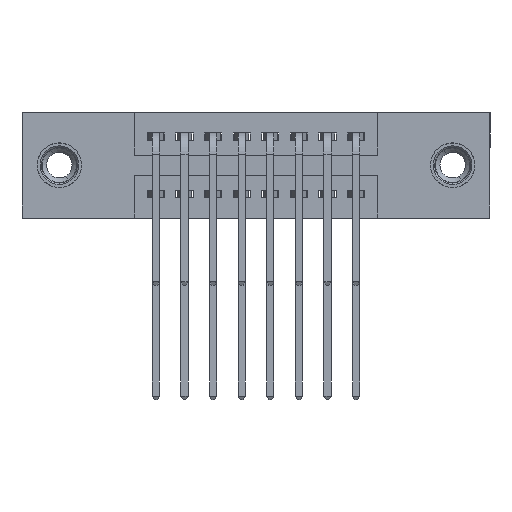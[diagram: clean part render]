
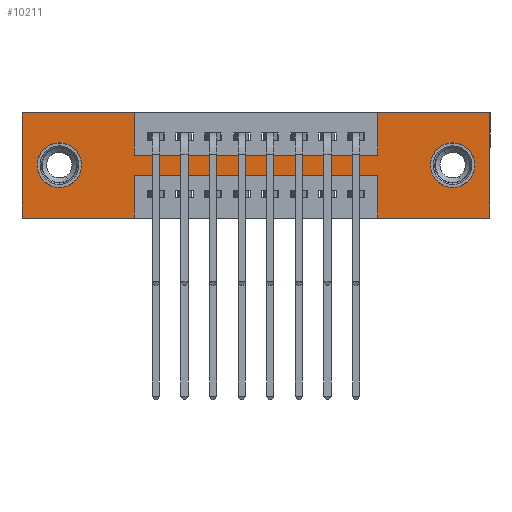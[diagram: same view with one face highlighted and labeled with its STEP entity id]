
A CAD part, front view. The second image highlights one B-rep face of the part: STEP entity #10211.
In plain terms, the highlighted planar face has unit normal (0, -1, 0).
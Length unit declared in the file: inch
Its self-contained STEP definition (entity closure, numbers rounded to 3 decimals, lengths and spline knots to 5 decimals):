
#52 = DIRECTION ( 'NONE',  ( 0., 1., 0. ) ) ;
#525 = DIRECTION ( 'NONE',  ( 0., 0., -1. ) ) ;
#569 = CARTESIAN_POINT ( 'NONE',  ( 0.3925, 0., -0.22 ) ) ;
#693 = AXIS2_PLACEMENT_3D ( 'NONE', #2639, #15776, #7985 ) ;
#1186 = DIRECTION ( 'NONE',  ( 0., 0., 1. ) ) ;
#1312 = DIRECTION ( 'NONE',  ( 0., 0., -1. ) ) ;
#1375 = CARTESIAN_POINT ( 'NONE',  ( 0.3925, 0., 0. ) ) ;
#1648 = CARTESIAN_POINT ( 'NONE',  ( 0., 0., 0. ) ) ;
#1840 = CARTESIAN_POINT ( 'NONE',  ( 1.635, 0., 0. ) ) ;
#1957 = ORIENTED_EDGE ( 'NONE', *, *, #4382, .F. ) ;
#1987 = VERTEX_POINT ( 'NONE', #11569 ) ;
#2229 = LINE ( 'NONE', #569, #15435 ) ;
#2528 = DIRECTION ( 'NONE',  ( -1., 0., 0. ) ) ;
#2639 = CARTESIAN_POINT ( 'NONE',  ( 0., 0., -0.37 ) ) ;
#2667 = CARTESIAN_POINT ( 'NONE',  ( 0.13, 0., -0.107 ) ) ;
#2683 = EDGE_CURVE ( 'NONE', #12558, #16761, #2229, .T. ) ;
#2698 = CARTESIAN_POINT ( 'NONE',  ( 1.635, 0., 0. ) ) ;
#2862 = CARTESIAN_POINT ( 'NONE',  ( 0.13, 0., -0.263 ) ) ;
#2925 = ORIENTED_EDGE ( 'NONE', *, *, #3582, .T. ) ;
#3055 = CIRCLE ( 'NONE', #13209, 0.078 ) ;
#3078 = EDGE_CURVE ( 'NONE', #12972, #1987, #13620, .T. ) ;
#3088 = VERTEX_POINT ( 'NONE', #1840 ) ;
#3273 = VECTOR ( 'NONE', #8458, 39.37008 ) ;
#3447 = VERTEX_POINT ( 'NONE', #5974 ) ;
#3582 = EDGE_CURVE ( 'NONE', #11357, #16199, #3055, .T. ) ;
#3595 = CARTESIAN_POINT ( 'NONE',  ( 1.505, 0., -0.185 ) ) ;
#3670 = ORIENTED_EDGE ( 'NONE', *, *, #4108, .F. ) ;
#3720 = LINE ( 'NONE', #15679, #3273 ) ;
#3743 = VERTEX_POINT ( 'NONE', #10683 ) ;
#3800 = EDGE_CURVE ( 'NONE', #5296, #11635, #3720, .T. ) ;
#3834 = CARTESIAN_POINT ( 'NONE',  ( 0.13, 0., -0.185 ) ) ;
#4108 = EDGE_CURVE ( 'NONE', #15454, #5059, #12794, .T. ) ;
#4382 = EDGE_CURVE ( 'NONE', #11635, #12558, #5559, .T. ) ;
#4551 = FACE_BOUND ( 'NONE', #7735, .T. ) ;
#4622 = LINE ( 'NONE', #15561, #17249 ) ;
#4945 = EDGE_CURVE ( 'NONE', #16761, #15454, #5152, .T. ) ;
#4949 = ORIENTED_EDGE ( 'NONE', *, *, #16121, .F. ) ;
#5027 = CARTESIAN_POINT ( 'NONE',  ( 0.3925, 0., -0.37 ) ) ;
#5059 = VERTEX_POINT ( 'NONE', #16961 ) ;
#5152 = LINE ( 'NONE', #5027, #15149 ) ;
#5187 = DIRECTION ( 'NONE',  ( 0., 0., 1. ) ) ;
#5254 = CARTESIAN_POINT ( 'NONE',  ( 0.3925, 0., -0.15 ) ) ;
#5296 = VERTEX_POINT ( 'NONE', #7044 ) ;
#5333 = DIRECTION ( 'NONE',  ( 0., 0., 1. ) ) ;
#5516 = CIRCLE ( 'NONE', #12430, 0.078 ) ;
#5559 = LINE ( 'NONE', #5957, #9507 ) ;
#5634 = CARTESIAN_POINT ( 'NONE',  ( 0.3925, 0., 0. ) ) ;
#5675 = CARTESIAN_POINT ( 'NONE',  ( 0., 0., 0. ) ) ;
#5957 = CARTESIAN_POINT ( 'NONE',  ( 1.2425, 0., -0.37 ) ) ;
#5974 = CARTESIAN_POINT ( 'NONE',  ( 1.2425, 0., -0.15 ) ) ;
#6252 = ORIENTED_EDGE ( 'NONE', *, *, #16261, .F. ) ;
#6683 = VERTEX_POINT ( 'NONE', #9461 ) ;
#6778 = VERTEX_POINT ( 'NONE', #5254 ) ;
#6983 = DIRECTION ( 'NONE',  ( 1., 0., 0. ) ) ;
#7044 = CARTESIAN_POINT ( 'NONE',  ( 1.635, 0., -0.37 ) ) ;
#7066 = DIRECTION ( 'NONE',  ( 0., 0., 1. ) ) ;
#7103 = LINE ( 'NONE', #5675, #16699 ) ;
#7325 = ORIENTED_EDGE ( 'NONE', *, *, #9291, .F. ) ;
#7330 = CIRCLE ( 'NONE', #9823, 0.078 ) ;
#7569 = VERTEX_POINT ( 'NONE', #5634 ) ;
#7679 = LINE ( 'NONE', #1375, #10777 ) ;
#7689 = VECTOR ( 'NONE', #13146, 39.37008 ) ;
#7735 = EDGE_LOOP ( 'NONE', ( #2925, #8733 ) ) ;
#7772 = DIRECTION ( 'NONE',  ( 0., 0., -1. ) ) ;
#7925 = PLANE ( 'NONE',  #693 ) ;
#7985 = DIRECTION ( 'NONE',  ( 0., 0., -1. ) ) ;
#7991 = EDGE_CURVE ( 'NONE', #6683, #7569, #4622, .T. ) ;
#8433 = DIRECTION ( 'NONE',  ( 0., 1., 0. ) ) ;
#8444 = LINE ( 'NONE', #10135, #14968 ) ;
#8458 = DIRECTION ( 'NONE',  ( -1., 0., 0. ) ) ;
#8558 = DIRECTION ( 'NONE',  ( -1., 0., 0. ) ) ;
#8690 = DIRECTION ( 'NONE',  ( 0., 1., 0. ) ) ;
#8716 = EDGE_CURVE ( 'NONE', #3447, #3743, #12024, .T. ) ;
#8733 = ORIENTED_EDGE ( 'NONE', *, *, #16025, .T. ) ;
#9291 = EDGE_CURVE ( 'NONE', #7569, #6778, #7679, .T. ) ;
#9461 = CARTESIAN_POINT ( 'NONE',  ( 0., 0., 0. ) ) ;
#9507 = VECTOR ( 'NONE', #1186, 39.37008 ) ;
#9724 = VECTOR ( 'NONE', #8558, 39.37008 ) ;
#9823 = AXIS2_PLACEMENT_3D ( 'NONE', #3834, #13061, #5187 ) ;
#9898 = ORIENTED_EDGE ( 'NONE', *, *, #7991, .F. ) ;
#10037 = AXIS2_PLACEMENT_3D ( 'NONE', #3595, #8433, #7772 ) ;
#10122 = VECTOR ( 'NONE', #7066, 39.37008 ) ;
#10135 = CARTESIAN_POINT ( 'NONE',  ( 0.3925, 0., -0.15 ) ) ;
#10211 = ADVANCED_FACE ( 'NONE', ( #11153, #4551, #14982 ), #7925, .T. ) ;
#10221 = CARTESIAN_POINT ( 'NONE',  ( 0.3925, 0., -0.37 ) ) ;
#10429 = DIRECTION ( 'NONE',  ( 1., 0., 0. ) ) ;
#10627 = EDGE_CURVE ( 'NONE', #6778, #3447, #8444, .T. ) ;
#10658 = DIRECTION ( 'NONE',  ( 0., 0., -1. ) ) ;
#10683 = CARTESIAN_POINT ( 'NONE',  ( 1.2425, 0., 0. ) ) ;
#10777 = VECTOR ( 'NONE', #1312, 39.37008 ) ;
#11153 = FACE_BOUND ( 'NONE', #11167, .T. ) ;
#11167 = EDGE_LOOP ( 'NONE', ( #14946, #13212 ) ) ;
#11333 = CARTESIAN_POINT ( 'NONE',  ( 1.505, 0., -0.107 ) ) ;
#11357 = VERTEX_POINT ( 'NONE', #2667 ) ;
#11429 = DIRECTION ( 'NONE',  ( 1., 0., 0. ) ) ;
#11561 = ORIENTED_EDGE ( 'NONE', *, *, #11589, .F. ) ;
#11569 = CARTESIAN_POINT ( 'NONE',  ( 1.505, 0., -0.263 ) ) ;
#11589 = EDGE_CURVE ( 'NONE', #5059, #6683, #13574, .T. ) ;
#11635 = VERTEX_POINT ( 'NONE', #16233 ) ;
#11725 = ORIENTED_EDGE ( 'NONE', *, *, #8716, .F. ) ;
#11830 = CARTESIAN_POINT ( 'NONE',  ( 1.2425, 0., 0. ) ) ;
#11890 = CARTESIAN_POINT ( 'NONE',  ( 0.3925, 0., -0.22 ) ) ;
#12024 = LINE ( 'NONE', #11830, #7689 ) ;
#12269 = LINE ( 'NONE', #2698, #15690 ) ;
#12430 = AXIS2_PLACEMENT_3D ( 'NONE', #16456, #8690, #525 ) ;
#12558 = VERTEX_POINT ( 'NONE', #17050 ) ;
#12794 = LINE ( 'NONE', #13662, #9724 ) ;
#12937 = EDGE_CURVE ( 'NONE', #1987, #12972, #5516, .T. ) ;
#12972 = VERTEX_POINT ( 'NONE', #11333 ) ;
#13061 = DIRECTION ( 'NONE',  ( 0., 1., 0. ) ) ;
#13146 = DIRECTION ( 'NONE',  ( 0., 0., 1. ) ) ;
#13205 = EDGE_LOOP ( 'NONE', ( #14039, #14312, #1957, #15871, #4949, #6252, #11725, #16828, #7325, #9898, #11561, #3670 ) ) ;
#13209 = AXIS2_PLACEMENT_3D ( 'NONE', #15483, #52, #5333 ) ;
#13212 = ORIENTED_EDGE ( 'NONE', *, *, #12937, .T. ) ;
#13574 = LINE ( 'NONE', #1648, #10122 ) ;
#13620 = CIRCLE ( 'NONE', #10037, 0.078 ) ;
#13662 = CARTESIAN_POINT ( 'NONE',  ( 0., 0., -0.37 ) ) ;
#14039 = ORIENTED_EDGE ( 'NONE', *, *, #4945, .F. ) ;
#14312 = ORIENTED_EDGE ( 'NONE', *, *, #2683, .F. ) ;
#14946 = ORIENTED_EDGE ( 'NONE', *, *, #3078, .T. ) ;
#14968 = VECTOR ( 'NONE', #11429, 39.37008 ) ;
#14982 = FACE_OUTER_BOUND ( 'NONE', #13205, .T. ) ;
#15149 = VECTOR ( 'NONE', #16757, 39.37008 ) ;
#15435 = VECTOR ( 'NONE', #2528, 39.37008 ) ;
#15454 = VERTEX_POINT ( 'NONE', #10221 ) ;
#15483 = CARTESIAN_POINT ( 'NONE',  ( 0.13, 0., -0.185 ) ) ;
#15561 = CARTESIAN_POINT ( 'NONE',  ( 0., 0., 0. ) ) ;
#15679 = CARTESIAN_POINT ( 'NONE',  ( 0., 0., -0.37 ) ) ;
#15690 = VECTOR ( 'NONE', #10658, 39.37008 ) ;
#15776 = DIRECTION ( 'NONE',  ( 0., -1., 0. ) ) ;
#15871 = ORIENTED_EDGE ( 'NONE', *, *, #3800, .F. ) ;
#16025 = EDGE_CURVE ( 'NONE', #16199, #11357, #7330, .T. ) ;
#16121 = EDGE_CURVE ( 'NONE', #3088, #5296, #12269, .T. ) ;
#16199 = VERTEX_POINT ( 'NONE', #2862 ) ;
#16233 = CARTESIAN_POINT ( 'NONE',  ( 1.2425, 0., -0.37 ) ) ;
#16261 = EDGE_CURVE ( 'NONE', #3743, #3088, #7103, .T. ) ;
#16456 = CARTESIAN_POINT ( 'NONE',  ( 1.505, 0., -0.185 ) ) ;
#16699 = VECTOR ( 'NONE', #6983, 39.37008 ) ;
#16757 = DIRECTION ( 'NONE',  ( 0., 0., -1. ) ) ;
#16761 = VERTEX_POINT ( 'NONE', #11890 ) ;
#16828 = ORIENTED_EDGE ( 'NONE', *, *, #10627, .F. ) ;
#16961 = CARTESIAN_POINT ( 'NONE',  ( 0., 0., -0.37 ) ) ;
#17050 = CARTESIAN_POINT ( 'NONE',  ( 1.2425, 0., -0.22 ) ) ;
#17249 = VECTOR ( 'NONE', #10429, 39.37008 ) ;
